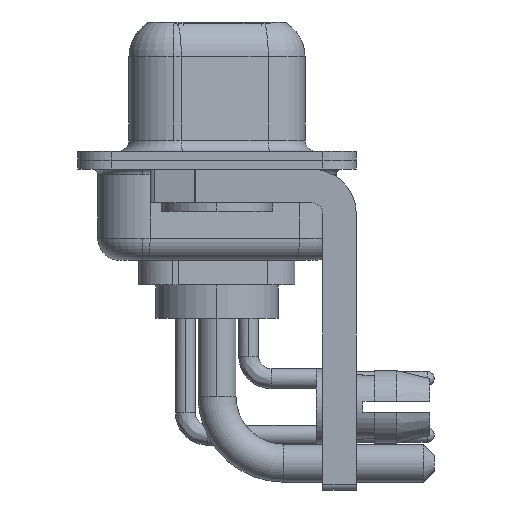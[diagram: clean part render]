
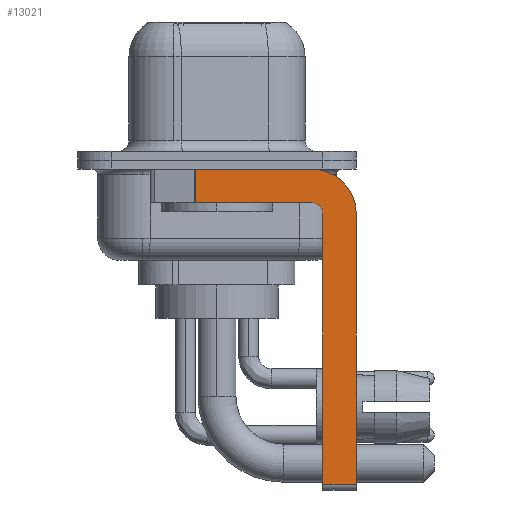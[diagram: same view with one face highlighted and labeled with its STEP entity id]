
A CAD part, left-side view. The second image highlights one B-rep face of the part: STEP entity #13021.
In plain terms, the highlighted planar face has unit normal (-1, 0, 0).
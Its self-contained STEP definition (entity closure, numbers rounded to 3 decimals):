
#276 = ORIENTED_EDGE ( 'NONE', *, *, #3755, .F. ) ;
#446 = EDGE_CURVE ( 'NONE', #17765, #13885, #4466, .T. ) ;
#1379 = EDGE_CURVE ( 'NONE', #17765, #15778, #17768, .T. ) ;
#1744 = VECTOR ( 'NONE', #14712, 1000. ) ;
#1844 = ORIENTED_EDGE ( 'NONE', *, *, #7183, .F. ) ;
#2448 = DIRECTION ( 'NONE',  ( 0., 0., -1. ) ) ;
#2552 = VECTOR ( 'NONE', #3150, 1000. ) ;
#2731 = ORIENTED_EDGE ( 'NONE', *, *, #18250, .F. ) ;
#3109 = CARTESIAN_POINT ( 'NONE',  ( -2.9, -6.25, -2.4 ) ) ;
#3150 = DIRECTION ( 'NONE',  ( 0., -1., 0. ) ) ;
#3447 = VECTOR ( 'NONE', #8577, 1000. ) ;
#3558 = CARTESIAN_POINT ( 'NONE',  ( -2.9, 0.978, -1.9 ) ) ;
#3708 = VECTOR ( 'NONE', #10891, 1000. ) ;
#3755 = EDGE_CURVE ( 'NONE', #7372, #14163, #14234, .T. ) ;
#4101 = ORIENTED_EDGE ( 'NONE', *, *, #446, .F. ) ;
#4466 = LINE ( 'NONE', #10415, #3447 ) ;
#4933 = CARTESIAN_POINT ( 'NONE',  ( -2.9, -4.25, -2.4 ) ) ;
#4982 = CARTESIAN_POINT ( 'NONE',  ( -2.9, 0.978, -1.9 ) ) ;
#5753 = ORIENTED_EDGE ( 'NONE', *, *, #18199, .F. ) ;
#6414 = LINE ( 'NONE', #16741, #3708 ) ;
#6966 = VECTOR ( 'NONE', #18509, 1000. ) ;
#7183 = EDGE_CURVE ( 'NONE', #14913, #11969, #6414, .T. ) ;
#7372 = VERTEX_POINT ( 'NONE', #17595 ) ;
#7473 = PLANE ( 'NONE',  #10969 ) ;
#7662 = ORIENTED_EDGE ( 'NONE', *, *, #1379, .T. ) ;
#8050 = DIRECTION ( 'NONE',  ( 0., 0., -1. ) ) ;
#8577 = DIRECTION ( 'NONE',  ( 0., 0., 1. ) ) ;
#8851 = FACE_OUTER_BOUND ( 'NONE', #11676, .T. ) ;
#8984 = ORIENTED_EDGE ( 'NONE', *, *, #10932, .F. ) ;
#9342 = CIRCLE ( 'NONE', #15859, 2. ) ;
#9872 = ORIENTED_EDGE ( 'NONE', *, *, #11887, .T. ) ;
#9934 = CARTESIAN_POINT ( 'NONE',  ( -2.9, -4.25, -1.9 ) ) ;
#10415 = CARTESIAN_POINT ( 'NONE',  ( -2.9, -4.75, -14.8 ) ) ;
#10462 = AXIS2_PLACEMENT_3D ( 'NONE', #4933, #14909, #12087 ) ;
#10503 = DIRECTION ( 'NONE',  ( 1., 0., 0. ) ) ;
#10891 = DIRECTION ( 'NONE',  ( 0., -1., 0. ) ) ;
#10932 = EDGE_CURVE ( 'NONE', #11969, #13400, #9342, .T. ) ;
#10969 = AXIS2_PLACEMENT_3D ( 'NONE', #13424, #10503, #18001 ) ;
#11230 = CARTESIAN_POINT ( 'NONE',  ( -2.9, -4.25, -2.4 ) ) ;
#11676 = EDGE_LOOP ( 'NONE', ( #1844, #9872, #276, #5753, #4101, #7662, #2731, #8984 ) ) ;
#11887 = EDGE_CURVE ( 'NONE', #14913, #14163, #15272, .T. ) ;
#11969 = VERTEX_POINT ( 'NONE', #12997 ) ;
#12087 = DIRECTION ( 'NONE',  ( 0., 0., 1. ) ) ;
#12997 = CARTESIAN_POINT ( 'NONE',  ( -2.9, -4.25, -0.4 ) ) ;
#13021 = ADVANCED_FACE ( 'NONE', ( #8851 ), #7473, .F. ) ;
#13081 = VECTOR ( 'NONE', #8050, 1000. ) ;
#13272 = CARTESIAN_POINT ( 'NONE',  ( -2.9, -4.75, -14.55 ) ) ;
#13400 = VERTEX_POINT ( 'NONE', #18656 ) ;
#13424 = CARTESIAN_POINT ( 'NONE',  ( -2.9, -4.25, -2.4 ) ) ;
#13451 = LINE ( 'NONE', #3109, #1744 ) ;
#13603 = CARTESIAN_POINT ( 'NONE',  ( -2.9, 0.978, -0.4 ) ) ;
#13885 = VERTEX_POINT ( 'NONE', #16201 ) ;
#14163 = VERTEX_POINT ( 'NONE', #4982 ) ;
#14234 = LINE ( 'NONE', #9934, #6966 ) ;
#14712 = DIRECTION ( 'NONE',  ( 0., 0., -1. ) ) ;
#14750 = CARTESIAN_POINT ( 'NONE',  ( -2.9, -4.25, -14.55 ) ) ;
#14909 = DIRECTION ( 'NONE',  ( -1., 0., 0. ) ) ;
#14913 = VERTEX_POINT ( 'NONE', #13603 ) ;
#15272 = LINE ( 'NONE', #3558, #13081 ) ;
#15778 = VERTEX_POINT ( 'NONE', #17374 ) ;
#15811 = DIRECTION ( 'NONE',  ( 1., 0., 0. ) ) ;
#15859 = AXIS2_PLACEMENT_3D ( 'NONE', #11230, #15811, #2448 ) ;
#16201 = CARTESIAN_POINT ( 'NONE',  ( -2.9, -4.75, -2.4 ) ) ;
#16741 = CARTESIAN_POINT ( 'NONE',  ( -2.9, 3., -0.4 ) ) ;
#17374 = CARTESIAN_POINT ( 'NONE',  ( -2.9, -6.25, -14.55 ) ) ;
#17595 = CARTESIAN_POINT ( 'NONE',  ( -2.9, -4.25, -1.9 ) ) ;
#17608 = CIRCLE ( 'NONE', #10462, 0.5 ) ;
#17765 = VERTEX_POINT ( 'NONE', #13272 ) ;
#17768 = LINE ( 'NONE', #14750, #2552 ) ;
#18001 = DIRECTION ( 'NONE',  ( 0., 0., -1. ) ) ;
#18199 = EDGE_CURVE ( 'NONE', #13885, #7372, #17608, .T. ) ;
#18250 = EDGE_CURVE ( 'NONE', #13400, #15778, #13451, .T. ) ;
#18509 = DIRECTION ( 'NONE',  ( 0., 1., 0. ) ) ;
#18656 = CARTESIAN_POINT ( 'NONE',  ( -2.9, -6.25, -2.4 ) ) ;
